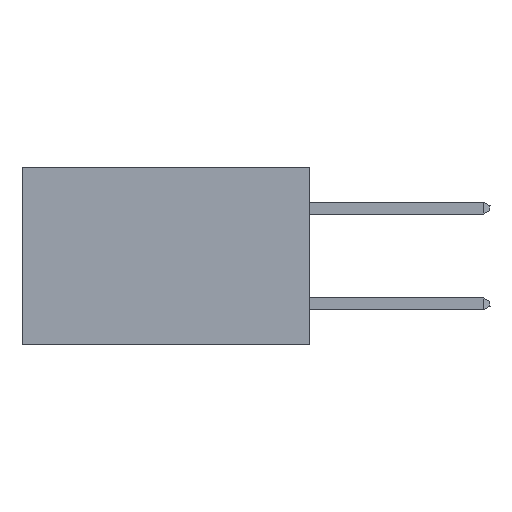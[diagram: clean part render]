
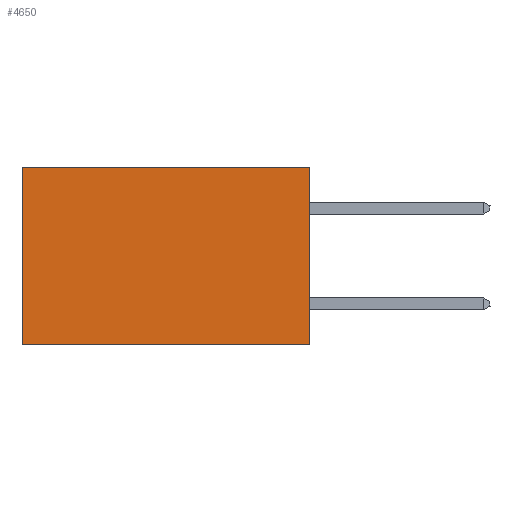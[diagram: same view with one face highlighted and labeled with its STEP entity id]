
A CAD part, left-side view. The second image highlights one B-rep face of the part: STEP entity #4650.
In plain terms, the highlighted planar face has unit normal (-1, 0, 0).
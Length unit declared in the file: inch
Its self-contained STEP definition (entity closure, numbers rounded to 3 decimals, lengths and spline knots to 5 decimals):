
#1322 = EDGE_CURVE ( 'NONE', #25848, #32782, #17076, .T. ) ;
#1950 = DIRECTION ( 'NONE',  ( 0., 0., -1. ) ) ;
#2533 = ORIENTED_EDGE ( 'NONE', *, *, #1322, .F. ) ;
#3721 = CARTESIAN_POINT ( 'NONE',  ( 0.2875, 0.6, 0. ) ) ;
#4650 = ADVANCED_FACE ( 'NONE', ( #29433 ), #19804, .F. ) ;
#5209 = CARTESIAN_POINT ( 'NONE',  ( 0.2875, 0., 0. ) ) ;
#6765 = AXIS2_PLACEMENT_3D ( 'NONE', #34374, #28832, #37162 ) ;
#7099 = CARTESIAN_POINT ( 'NONE',  ( 0.2875, 0., 0. ) ) ;
#7970 = EDGE_CURVE ( 'NONE', #25848, #14961, #34396, .T. ) ;
#9439 = LINE ( 'NONE', #16706, #27927 ) ;
#11264 = DIRECTION ( 'NONE',  ( 0., 1., 0. ) ) ;
#13495 = CARTESIAN_POINT ( 'NONE',  ( 0.2875, 0.6, 0. ) ) ;
#14961 = VERTEX_POINT ( 'NONE', #3721 ) ;
#16397 = DIRECTION ( 'NONE',  ( 0., 0., -1. ) ) ;
#16706 = CARTESIAN_POINT ( 'NONE',  ( 0.2875, 0., -0.37 ) ) ;
#17076 = LINE ( 'NONE', #5209, #19800 ) ;
#17382 = VECTOR ( 'NONE', #16397, 39.37008 ) ;
#17508 = ORIENTED_EDGE ( 'NONE', *, *, #24369, .F. ) ;
#18277 = LINE ( 'NONE', #13495, #17382 ) ;
#19090 = VECTOR ( 'NONE', #27208, 39.37008 ) ;
#19800 = VECTOR ( 'NONE', #1950, 39.37008 ) ;
#19804 = PLANE ( 'NONE',  #6765 ) ;
#20460 = EDGE_CURVE ( 'NONE', #14961, #26379, #18277, .T. ) ;
#24369 = EDGE_CURVE ( 'NONE', #32782, #26379, #9439, .T. ) ;
#25848 = VERTEX_POINT ( 'NONE', #29534 ) ;
#26379 = VERTEX_POINT ( 'NONE', #31211 ) ;
#27208 = DIRECTION ( 'NONE',  ( 0., 1., 0. ) ) ;
#27927 = VECTOR ( 'NONE', #11264, 39.37008 ) ;
#28832 = DIRECTION ( 'NONE',  ( 1., 0., 0. ) ) ;
#29031 = ORIENTED_EDGE ( 'NONE', *, *, #20460, .T. ) ;
#29433 = FACE_OUTER_BOUND ( 'NONE', #31165, .T. ) ;
#29534 = CARTESIAN_POINT ( 'NONE',  ( 0.2875, 0., 0. ) ) ;
#31165 = EDGE_LOOP ( 'NONE', ( #29031, #17508, #2533, #33633 ) ) ;
#31211 = CARTESIAN_POINT ( 'NONE',  ( 0.2875, 0.6, -0.37 ) ) ;
#32782 = VERTEX_POINT ( 'NONE', #35066 ) ;
#33633 = ORIENTED_EDGE ( 'NONE', *, *, #7970, .T. ) ;
#34374 = CARTESIAN_POINT ( 'NONE',  ( 0.2875, 0., 0. ) ) ;
#34396 = LINE ( 'NONE', #7099, #19090 ) ;
#35066 = CARTESIAN_POINT ( 'NONE',  ( 0.2875, 0., -0.37 ) ) ;
#37162 = DIRECTION ( 'NONE',  ( 0., 0., -1. ) ) ;
